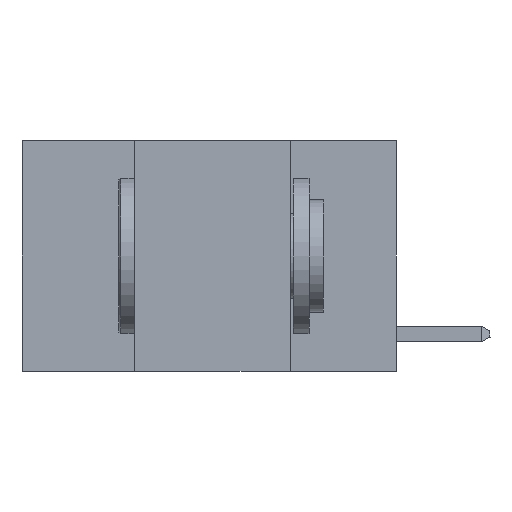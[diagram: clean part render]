
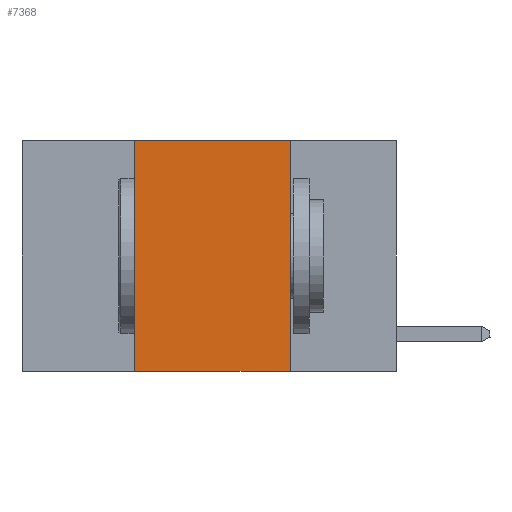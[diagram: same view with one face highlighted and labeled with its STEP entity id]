
A CAD part, left-side view. The second image highlights one B-rep face of the part: STEP entity #7368.
In plain terms, the highlighted planar face has unit normal (-1, 0, 0).
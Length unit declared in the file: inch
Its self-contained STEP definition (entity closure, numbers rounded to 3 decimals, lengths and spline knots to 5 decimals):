
#1436 = CARTESIAN_POINT ( 'NONE',  ( 0., 0.42, 0. ) ) ;
#1830 = VECTOR ( 'NONE', #3307, 39.37008 ) ;
#2058 = PLANE ( 'NONE',  #6216 ) ;
#2410 = EDGE_CURVE ( 'NONE', #9332, #2939, #13018, .T. ) ;
#2670 = CARTESIAN_POINT ( 'NONE',  ( 0., 0.42, 0. ) ) ;
#2939 = VERTEX_POINT ( 'NONE', #2670 ) ;
#3140 = DIRECTION ( 'NONE',  ( 1., 0., 0. ) ) ;
#3307 = DIRECTION ( 'NONE',  ( 0., -1., 0. ) ) ;
#3967 = CARTESIAN_POINT ( 'NONE',  ( 0., 0.17, 0. ) ) ;
#4195 = VERTEX_POINT ( 'NONE', #13841 ) ;
#4267 = EDGE_CURVE ( 'NONE', #9538, #4195, #9563, .T. ) ;
#4393 = LINE ( 'NONE', #14797, #12141 ) ;
#4462 = DIRECTION ( 'NONE',  ( 0., -1., 0. ) ) ;
#4509 = CARTESIAN_POINT ( 'NONE',  ( 0., 0.6, 0. ) ) ;
#4532 = LINE ( 'NONE', #13953, #1830 ) ;
#4856 = CARTESIAN_POINT ( 'NONE',  ( 0., 0.17, 0. ) ) ;
#5415 = VECTOR ( 'NONE', #9577, 39.37008 ) ;
#5537 = ORIENTED_EDGE ( 'NONE', *, *, #4267, .F. ) ;
#6216 = AXIS2_PLACEMENT_3D ( 'NONE', #4509, #3140, #12767 ) ;
#6720 = CARTESIAN_POINT ( 'NONE',  ( 0., 0.42, -0.37 ) ) ;
#7368 = ADVANCED_FACE ( 'NONE', ( #9271 ), #2058, .F. ) ;
#9095 = VECTOR ( 'NONE', #14223, 39.37008 ) ;
#9271 = FACE_OUTER_BOUND ( 'NONE', #13065, .T. ) ;
#9332 = VERTEX_POINT ( 'NONE', #6720 ) ;
#9538 = VERTEX_POINT ( 'NONE', #4856 ) ;
#9563 = LINE ( 'NONE', #3967, #9095 ) ;
#9577 = DIRECTION ( 'NONE',  ( 0., 0., 1. ) ) ;
#11032 = ORIENTED_EDGE ( 'NONE', *, *, #12857, .F. ) ;
#11138 = EDGE_CURVE ( 'NONE', #9332, #4195, #4532, .T. ) ;
#12141 = VECTOR ( 'NONE', #4462, 39.37008 ) ;
#12272 = ORIENTED_EDGE ( 'NONE', *, *, #2410, .F. ) ;
#12507 = ORIENTED_EDGE ( 'NONE', *, *, #11138, .T. ) ;
#12767 = DIRECTION ( 'NONE',  ( 0., 0., -1. ) ) ;
#12857 = EDGE_CURVE ( 'NONE', #2939, #9538, #4393, .T. ) ;
#13018 = LINE ( 'NONE', #1436, #5415 ) ;
#13065 = EDGE_LOOP ( 'NONE', ( #5537, #11032, #12272, #12507 ) ) ;
#13841 = CARTESIAN_POINT ( 'NONE',  ( 0., 0.17, -0.37 ) ) ;
#13953 = CARTESIAN_POINT ( 'NONE',  ( 0., 0.6, -0.37 ) ) ;
#14223 = DIRECTION ( 'NONE',  ( 0., 0., -1. ) ) ;
#14797 = CARTESIAN_POINT ( 'NONE',  ( 0., 0.6, 0. ) ) ;
